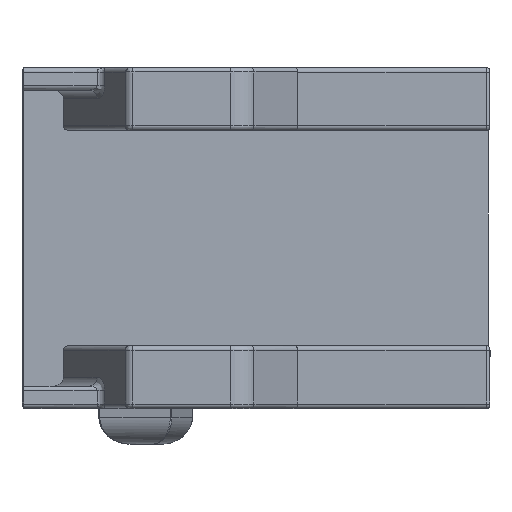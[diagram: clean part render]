
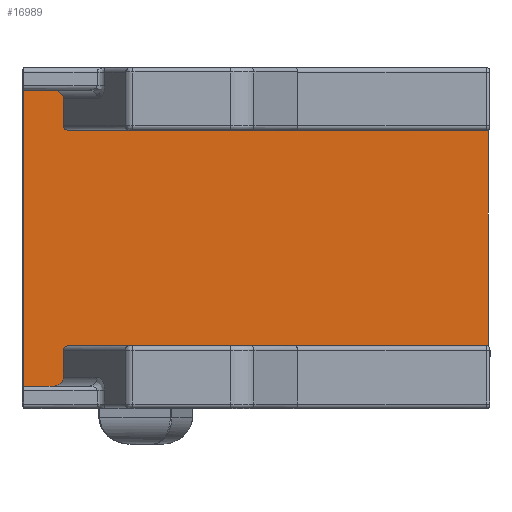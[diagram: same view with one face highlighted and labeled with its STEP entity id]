
A CAD part, left-side view. The second image highlights one B-rep face of the part: STEP entity #16989.
In plain terms, the highlighted planar face has unit normal (-1, 0, 0).
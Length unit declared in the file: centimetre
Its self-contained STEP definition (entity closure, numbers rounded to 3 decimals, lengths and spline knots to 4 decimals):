
#336=PLANE($,#18201);
#2015=LINE($,#30475,#3136);
#2027=LINE($,#30504,#3148);
#2069=LINE($,#30881,#3190);
#2086=LINE($,#31112,#3207);
#2129=LINE($,#31230,#3250);
#2281=LINE($,#32494,#3402);
#2290=LINE($,#32594,#3411);
#2680=LINE($,#37543,#3801);
#3136=VECTOR($,#19170,3.3);
#3148=VECTOR($,#19204,0.3263);
#3190=VECTOR($,#19296,2.48);
#3207=VECTOR($,#19385,4.6385);
#3250=VECTOR($,#19456,4.6385);
#3402=VECTOR($,#19886,0.3);
#3411=VECTOR($,#19919,0.3);
#3801=VECTOR($,#21713,0.3263);
#3853=ELLIPSE($,#17302,0.0402,0.04);
#3860=ELLIPSE($,#17326,0.0402,0.04);
#3879=ELLIPSE($,#17503,0.0577,0.05);
#3880=ELLIPSE($,#17518,0.0577,0.05);
#3881=ELLIPSE($,#17520,0.1155,0.1);
#3882=ELLIPSE($,#17523,0.1155,0.1);
#5288=FACE_OUTER_BOUND($,#6319,.T.);
#6319=EDGE_LOOP($,(#15898,#15899,#15900,#15901,#15902,#15903,#15904,#15905,
#15906,#15907,#15908,#15909,#15910,#15911));
#7555=VERTEX_POINT($,#30436);
#7563=VERTEX_POINT($,#30471);
#7569=VERTEX_POINT($,#30502);
#7613=VERTEX_POINT($,#30879);
#7614=VERTEX_POINT($,#30880);
#7628=VERTEX_POINT($,#30910);
#7636=VERTEX_POINT($,#31096);
#7642=VERTEX_POINT($,#31110);
#7683=VERTEX_POINT($,#31229);
#7817=VERTEX_POINT($,#32491);
#7818=VERTEX_POINT($,#32493);
#7824=VERTEX_POINT($,#32585);
#7827=VERTEX_POINT($,#32592);
#7831=VERTEX_POINT($,#32646);
#9504=EDGE_CURVE($,#7555,#7563,#2015,.T.);
#9519=EDGE_CURVE($,#7569,#7555,#2027,.T.);
#9589=EDGE_CURVE($,#7613,#7614,#2069,.T.);
#9604=EDGE_CURVE($,#7613,#7628,#3853,.F.);
#9626=EDGE_CURVE($,#7636,#7614,#3860,.F.);
#9634=EDGE_CURVE($,#7642,#7636,#2086,.T.);
#9684=EDGE_CURVE($,#7628,#7683,#2129,.T.);
#9928=EDGE_CURVE($,#7818,#7817,#2281,.T.);
#9944=EDGE_CURVE($,#7824,#7827,#2290,.T.);
#9953=EDGE_CURVE($,#7683,#7817,#3879,.F.);
#9961=EDGE_CURVE($,#7824,#7642,#3880,.F.);
#9962=EDGE_CURVE($,#7827,#7831,#3881,.T.);
#9965=EDGE_CURVE($,#7569,#7818,#3882,.T.);
#10865=EDGE_CURVE($,#7563,#7831,#2680,.T.);
#15898=ORIENTED_EDGE($,*,*,#9504,.F.);
#15899=ORIENTED_EDGE($,*,*,#9519,.F.);
#15900=ORIENTED_EDGE($,*,*,#9965,.T.);
#15901=ORIENTED_EDGE($,*,*,#9928,.T.);
#15902=ORIENTED_EDGE($,*,*,#9953,.F.);
#15903=ORIENTED_EDGE($,*,*,#9684,.F.);
#15904=ORIENTED_EDGE($,*,*,#9604,.F.);
#15905=ORIENTED_EDGE($,*,*,#9589,.T.);
#15906=ORIENTED_EDGE($,*,*,#9626,.F.);
#15907=ORIENTED_EDGE($,*,*,#9634,.F.);
#15908=ORIENTED_EDGE($,*,*,#9961,.F.);
#15909=ORIENTED_EDGE($,*,*,#9944,.T.);
#15910=ORIENTED_EDGE($,*,*,#9962,.T.);
#15911=ORIENTED_EDGE($,*,*,#10865,.F.);
#16989=ADVANCED_FACE($,(#5288),#336,.F.);
#17302=AXIS2_PLACEMENT_3D($,#30911,#19320,#19321);
#17326=AXIS2_PLACEMENT_3D($,#31097,#19372,#19373);
#17503=AXIS2_PLACEMENT_3D($,#32611,#19941,#19942);
#17518=AXIS2_PLACEMENT_3D($,#32644,#19971,#19972);
#17520=AXIS2_PLACEMENT_3D($,#32647,#19975,#19976);
#17523=AXIS2_PLACEMENT_3D($,#32652,#19982,#19983);
#18201=AXIS2_PLACEMENT_3D($,#37551,#21725,#21726);
#19170=DIRECTION($,(0.,0.,1.));
#19204=DIRECTION($,(0.,1.,0.));
#19296=DIRECTION($,(0.,0.,1.));
#19320=DIRECTION('center_axis',(1.,0.,0.));
#19321=DIRECTION('ref_axis',(0.,-1.,0.));
#19372=DIRECTION('center_axis',(1.,0.,0.));
#19373=DIRECTION('ref_axis',(0.,-1.,0.));
#19385=DIRECTION($,(0.,-1.,0.));
#19456=DIRECTION($,(0.,1.,0.));
#19886=DIRECTION($,(0.,0.,1.));
#19919=DIRECTION($,(0.,0.,1.));
#19941=DIRECTION('center_axis',(1.,0.,0.));
#19942=DIRECTION('ref_axis',(0.,1.,0.));
#19971=DIRECTION('center_axis',(1.,0.,0.));
#19972=DIRECTION('ref_axis',(0.,1.,0.));
#19975=DIRECTION('center_axis',(-1.,0.,0.));
#19976=DIRECTION('ref_axis',(0.,-1.,0.));
#19982=DIRECTION('center_axis',(-1.,0.,0.));
#19983=DIRECTION('ref_axis',(0.,-1.,0.));
#21713=DIRECTION($,(0.,-1.,0.));
#21725=DIRECTION('center_axis',(1.,0.,0.));
#21726=DIRECTION('ref_axis',(0.,0.,-1.));
#30436=CARTESIAN_POINT('',(-8.24,-0.949,-1.55));
#30471=CARTESIAN_POINT('',(-8.24,-0.949,1.75));
#30475=CARTESIAN_POINT($,(-8.24,-0.949,0.0998));
#30502=CARTESIAN_POINT('',(-8.24,-1.2753,-1.55));
#30504=CARTESIAN_POINT($,(-8.24,-3.1547,-1.55));
#30879=CARTESIAN_POINT('',(-8.24,-6.1271,-1.14));
#30880=CARTESIAN_POINT('',(-8.24,-6.1271,1.34));
#30881=CARTESIAN_POINT($,(-8.24,-6.1271,0.1));
#30910=CARTESIAN_POINT('',(-8.24,-6.0869,-1.1));
#30911=CARTESIAN_POINT('Origin',(-8.24,-6.0869,-1.14));
#31096=CARTESIAN_POINT('',(-8.24,-6.0869,1.3));
#31097=CARTESIAN_POINT('Origin',(-8.24,-6.0869,1.34));
#31110=CARTESIAN_POINT('',(-8.24,-1.4485,1.3));
#31112=CARTESIAN_POINT($,(-8.24,-3.284,1.3));
#31229=CARTESIAN_POINT('',(-8.24,-1.4485,-1.1));
#31230=CARTESIAN_POINT($,(-8.24,-3.1547,-1.1));
#32491=CARTESIAN_POINT('',(-8.24,-1.3907,-1.15));
#32493=CARTESIAN_POINT('',(-8.24,-1.3907,-1.45));
#32494=CARTESIAN_POINT($,(-8.24,-1.3907,-0.91));
#32585=CARTESIAN_POINT('',(-8.24,-1.3907,1.35));
#32592=CARTESIAN_POINT('',(-8.24,-1.3907,1.65));
#32594=CARTESIAN_POINT($,(-8.24,-1.3907,-0.91));
#32611=CARTESIAN_POINT('Origin',(-8.24,-1.4485,-1.15));
#32644=CARTESIAN_POINT('Origin',(-8.24,-1.4485,1.35));
#32646=CARTESIAN_POINT('',(-8.24,-1.2753,1.75));
#32647=CARTESIAN_POINT('Origin',(-8.24,-1.2753,1.65));
#32652=CARTESIAN_POINT('Origin',(-8.24,-1.2753,-1.45));
#37543=CARTESIAN_POINT($,(-8.24,-3.284,1.75));
#37551=CARTESIAN_POINT('Origin',(-8.24,-3.1141,0.1));
